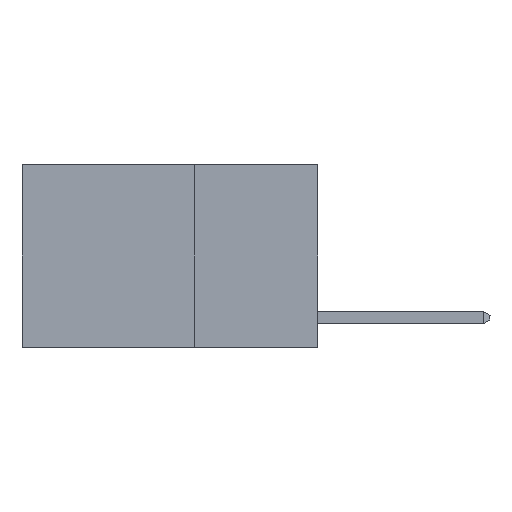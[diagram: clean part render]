
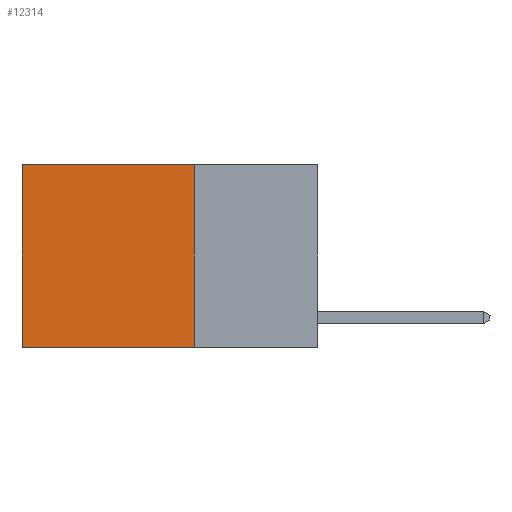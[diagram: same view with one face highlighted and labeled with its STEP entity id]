
A CAD part, left-side view. The second image highlights one B-rep face of the part: STEP entity #12314.
In plain terms, the highlighted planar face has unit normal (-1, 0, 0).
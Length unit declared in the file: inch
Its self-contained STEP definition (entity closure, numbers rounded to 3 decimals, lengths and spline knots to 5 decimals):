
#979 = CARTESIAN_POINT ( 'NONE',  ( 0.2625, 0.6, 0. ) ) ;
#3393 = CARTESIAN_POINT ( 'NONE',  ( 0.2625, 0.25, 0. ) ) ;
#3973 = DIRECTION ( 'NONE',  ( 0., 1., 0. ) ) ;
#4468 = CARTESIAN_POINT ( 'NONE',  ( 0.2625, 0.25, -0.37 ) ) ;
#6166 = VECTOR ( 'NONE', #3973, 39.37008 ) ;
#7031 = FACE_OUTER_BOUND ( 'NONE', #8194, .T. ) ;
#7569 = CARTESIAN_POINT ( 'NONE',  ( 0.2625, 0.25, 0. ) ) ;
#8194 = EDGE_LOOP ( 'NONE', ( #17131, #28608, #12505, #8738 ) ) ;
#8738 = ORIENTED_EDGE ( 'NONE', *, *, #12602, .T. ) ;
#11925 = VERTEX_POINT ( 'NONE', #4468 ) ;
#12314 = ADVANCED_FACE ( 'NONE', ( #7031 ), #20310, .F. ) ;
#12505 = ORIENTED_EDGE ( 'NONE', *, *, #26065, .F. ) ;
#12602 = EDGE_CURVE ( 'NONE', #17772, #26726, #17780, .T. ) ;
#12980 = DIRECTION ( 'NONE',  ( 0., 0., -1. ) ) ;
#12990 = DIRECTION ( 'NONE',  ( 0., 0., -1. ) ) ;
#13578 = CARTESIAN_POINT ( 'NONE',  ( 0.2625, 0.25, -0.37 ) ) ;
#14112 = EDGE_CURVE ( 'NONE', #11925, #16587, #24682, .T. ) ;
#14508 = DIRECTION ( 'NONE',  ( 0., 1., 0. ) ) ;
#15355 = VECTOR ( 'NONE', #12980, 39.37008 ) ;
#16587 = VERTEX_POINT ( 'NONE', #19958 ) ;
#17131 = ORIENTED_EDGE ( 'NONE', *, *, #22764, .T. ) ;
#17772 = VERTEX_POINT ( 'NONE', #7569 ) ;
#17780 = LINE ( 'NONE', #19360, #28066 ) ;
#19360 = CARTESIAN_POINT ( 'NONE',  ( 0.2625, 0.25, 0. ) ) ;
#19958 = CARTESIAN_POINT ( 'NONE',  ( 0.2625, 0.6, -0.37 ) ) ;
#20310 = PLANE ( 'NONE',  #20609 ) ;
#20609 = AXIS2_PLACEMENT_3D ( 'NONE', #3393, #27513, #12990 ) ;
#20730 = VECTOR ( 'NONE', #27902, 39.37008 ) ;
#21646 = LINE ( 'NONE', #979, #15355 ) ;
#21888 = LINE ( 'NONE', #27619, #20730 ) ;
#22764 = EDGE_CURVE ( 'NONE', #26726, #16587, #21646, .T. ) ;
#24682 = LINE ( 'NONE', #13578, #6166 ) ;
#25661 = CARTESIAN_POINT ( 'NONE',  ( 0.2625, 0.6, 0. ) ) ;
#26065 = EDGE_CURVE ( 'NONE', #17772, #11925, #21888, .T. ) ;
#26726 = VERTEX_POINT ( 'NONE', #25661 ) ;
#27513 = DIRECTION ( 'NONE',  ( 1., 0., 0. ) ) ;
#27619 = CARTESIAN_POINT ( 'NONE',  ( 0.2625, 0.25, 0. ) ) ;
#27902 = DIRECTION ( 'NONE',  ( 0., 0., -1. ) ) ;
#28066 = VECTOR ( 'NONE', #14508, 39.37008 ) ;
#28608 = ORIENTED_EDGE ( 'NONE', *, *, #14112, .F. ) ;
